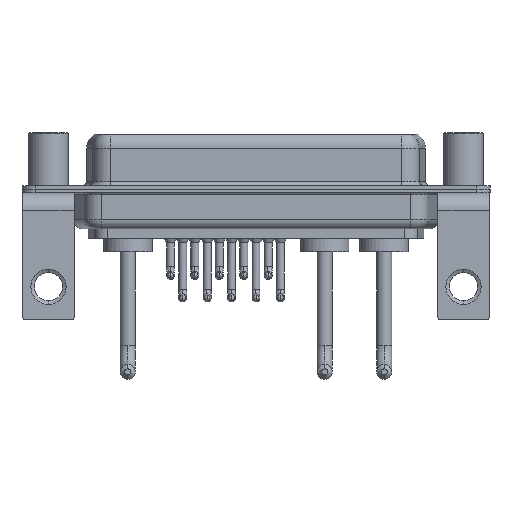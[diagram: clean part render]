
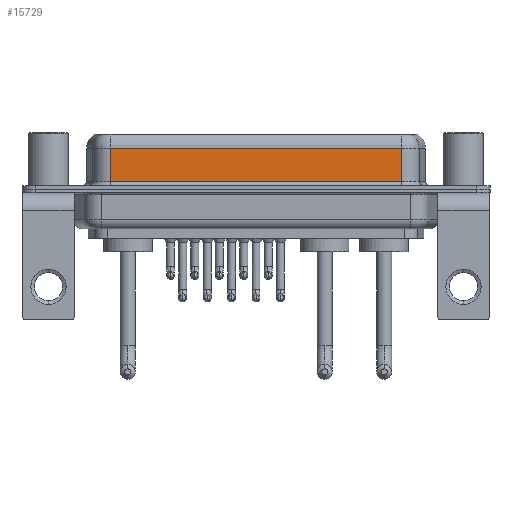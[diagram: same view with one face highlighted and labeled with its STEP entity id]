
A CAD part, front view. The second image highlights one B-rep face of the part: STEP entity #15729.
In plain terms, the highlighted planar face has unit normal (0, -1, 0).
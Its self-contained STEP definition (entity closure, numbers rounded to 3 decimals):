
#730 = ORIENTED_EDGE ( 'NONE', *, *, #20497, .T. ) ;
#1106 = ORIENTED_EDGE ( 'NONE', *, *, #15015, .F. ) ;
#1190 = VERTEX_POINT ( 'NONE', #6923 ) ;
#2874 = CARTESIAN_POINT ( 'NONE',  ( 7.013, -3.95, 0.9 ) ) ;
#3361 = ORIENTED_EDGE ( 'NONE', *, *, #6610, .T. ) ;
#4814 = DIRECTION ( 'NONE',  ( 0., 1., 0. ) ) ;
#6610 = EDGE_CURVE ( 'NONE', #8577, #1190, #11346, .T. ) ;
#6729 = DIRECTION ( 'NONE',  ( 0., 0., -1. ) ) ;
#6923 = CARTESIAN_POINT ( 'NONE',  ( 7.013, -3.95, 4.65 ) ) ;
#8577 = VERTEX_POINT ( 'NONE', #12177 ) ;
#9003 = ORIENTED_EDGE ( 'NONE', *, *, #20537, .T. ) ;
#9428 = VERTEX_POINT ( 'NONE', #2874 ) ;
#9995 = CARTESIAN_POINT ( 'NONE',  ( 40.037, -3.95, 6.4 ) ) ;
#10104 = DIRECTION ( 'NONE',  ( 1., 0., 0. ) ) ;
#11346 = LINE ( 'NONE', #12892, #17734 ) ;
#11756 = VECTOR ( 'NONE', #19857, 1000. ) ;
#11958 = LINE ( 'NONE', #18640, #13607 ) ;
#12177 = CARTESIAN_POINT ( 'NONE',  ( 40.037, -3.95, 4.65 ) ) ;
#12770 = EDGE_LOOP ( 'NONE', ( #1106, #3361, #9003, #730 ) ) ;
#12892 = CARTESIAN_POINT ( 'NONE',  ( 40.037, -3.95, 4.65 ) ) ;
#12904 = CARTESIAN_POINT ( 'NONE',  ( 40.037, -3.95, 6.4 ) ) ;
#13607 = VECTOR ( 'NONE', #6729, 1000. ) ;
#15015 = EDGE_CURVE ( 'NONE', #8577, #16033, #18311, .T. ) ;
#15729 = ADVANCED_FACE ( 'NONE', ( #17926 ), #19776, .F. ) ;
#16033 = VERTEX_POINT ( 'NONE', #17253 ) ;
#17008 = CARTESIAN_POINT ( 'NONE',  ( 40.037, -3.95, 0.9 ) ) ;
#17253 = CARTESIAN_POINT ( 'NONE',  ( 40.037, -3.95, 0.9 ) ) ;
#17734 = VECTOR ( 'NONE', #19552, 1000. ) ;
#17926 = FACE_OUTER_BOUND ( 'NONE', #12770, .T. ) ;
#18308 = LINE ( 'NONE', #17008, #20580 ) ;
#18311 = LINE ( 'NONE', #9995, #11756 ) ;
#18640 = CARTESIAN_POINT ( 'NONE',  ( 7.013, -3.95, 6.4 ) ) ;
#19552 = DIRECTION ( 'NONE',  ( -1., 0., 0. ) ) ;
#19562 = DIRECTION ( 'NONE',  ( 0., 0., 1. ) ) ;
#19776 = PLANE ( 'NONE',  #20166 ) ;
#19857 = DIRECTION ( 'NONE',  ( 0., 0., -1. ) ) ;
#20166 = AXIS2_PLACEMENT_3D ( 'NONE', #12904, #4814, #19562 ) ;
#20497 = EDGE_CURVE ( 'NONE', #9428, #16033, #18308, .T. ) ;
#20537 = EDGE_CURVE ( 'NONE', #1190, #9428, #11958, .T. ) ;
#20580 = VECTOR ( 'NONE', #10104, 1000. ) ;
